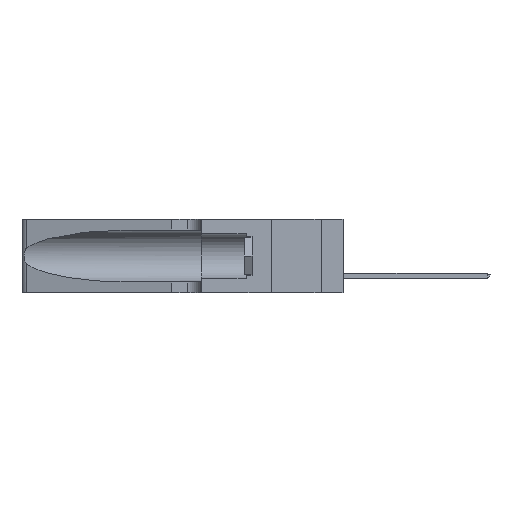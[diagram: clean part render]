
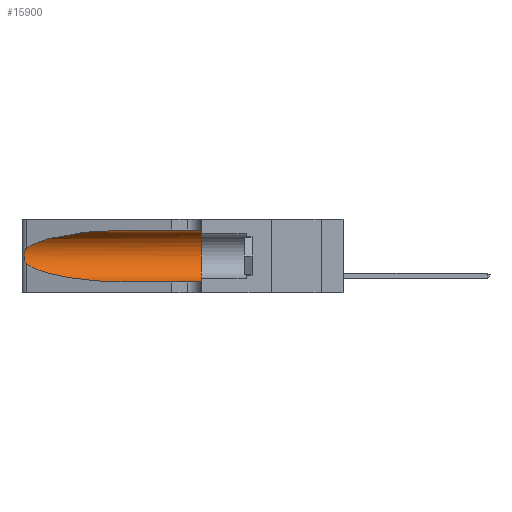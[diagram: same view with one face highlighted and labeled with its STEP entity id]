
A CAD part, left-side view. The second image highlights one B-rep face of the part: STEP entity #15900.
In plain terms, the highlighted cylindrical face has radius 3.308 mm (diameter 6.617 mm), a partial arc.
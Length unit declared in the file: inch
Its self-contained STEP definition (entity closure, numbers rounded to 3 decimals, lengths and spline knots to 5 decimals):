
#396 = CARTESIAN_POINT ( 'NONE',  ( 0.1305, 0.72297, 0.05475 ) ) ;
#763 = CARTESIAN_POINT ( 'NONE',  ( 0.25639, 1.23186, 0.15144 ) ) ;
#1344 = VERTEX_POINT ( 'NONE', #19258 ) ;
#3363 = ORIENTED_EDGE ( 'NONE', *, *, #23458, .F. ) ;
#3405 = CARTESIAN_POINT ( 'NONE',  ( 0.25555, 1.22994, 0.2215 ) ) ;
#3709 = ORIENTED_EDGE ( 'NONE', *, *, #23173, .T. ) ;
#3979 = CARTESIAN_POINT ( 'NONE',  ( 0.26018, 1.23835, 0.19895 ) ) ;
#4084 = CARTESIAN_POINT ( 'NONE',  ( 0.25856, 1.23593, 0.16098 ) ) ;
#5433 = CARTESIAN_POINT ( 'NONE',  ( 0.2373, 1.15595, 0.28018 ) ) ;
#5754 = LINE ( 'NONE', #24213, #10757 ) ;
#6524 = CARTESIAN_POINT ( 'NONE',  ( 0.1305, 0.35, 0.185 ) ) ;
#6635 = ORIENTED_EDGE ( 'NONE', *, *, #16826, .F. ) ;
#6646 = CARTESIAN_POINT ( 'NONE',  ( 0.26075, 1.23896, 0.19203 ) ) ;
#6819 = DIRECTION ( 'NONE',  ( 0., 1., 0. ) ) ;
#7966 = CARTESIAN_POINT ( 'NONE',  ( 0.1305, 1.61858, 0.31525 ) ) ;
#8261 = CARTESIAN_POINT ( 'NONE',  ( 0.25487, 1.22718, 0.14631 ) ) ;
#9195 = ORIENTED_EDGE ( 'NONE', *, *, #22257, .T. ) ;
#10757 = VECTOR ( 'NONE', #29354, 39.37008 ) ;
#12467 =( BOUNDED_CURVE ( )  B_SPLINE_CURVE ( 3, ( #27745, #15193, #5433, #30025 ),
 .UNSPECIFIED., .F., .F. ) 
 B_SPLINE_CURVE_WITH_KNOTS ( ( 4, 4 ),
 ( 1.5708, 2.84003 ),
 .UNSPECIFIED. ) 
 CURVE ( )  GEOMETRIC_REPRESENTATION_ITEM ( )  RATIONAL_B_SPLINE_CURVE ( ( 1., 0.87, 0.87, 1. ) ) 
 REPRESENTATION_ITEM ( '' )  );
#13260 = CARTESIAN_POINT ( 'NONE',  ( 0.2373, 1.15595, 0.08982 ) ) ;
#14399 = EDGE_CURVE ( 'NONE', #31760, #21525, #14988, .T. ) ;
#14880 = CARTESIAN_POINT ( 'NONE',  ( 0.25487, 1.22718, 0.14631 ) ) ;
#14988 =( BOUNDED_CURVE ( )  B_SPLINE_CURVE ( 3, ( #27934, #13260, #20321, #28037 ),
 .UNSPECIFIED., .F., .F. ) 
 B_SPLINE_CURVE_WITH_KNOTS ( ( 4, 4 ),
 ( 3.44316, 4.71239 ),
 .UNSPECIFIED. ) 
 CURVE ( )  GEOMETRIC_REPRESENTATION_ITEM ( )  RATIONAL_B_SPLINE_CURVE ( ( 1., 0.87, 0.87, 1. ) ) 
 REPRESENTATION_ITEM ( '' )  );
#15193 = CARTESIAN_POINT ( 'NONE',  ( 0.18966, 0.96281, 0.31525 ) ) ;
#15900 = ADVANCED_FACE ( 'NONE', ( #16791 ), #21415, .F. ) ;
#16285 = CARTESIAN_POINT ( 'NONE',  ( 0.26017, 1.23833, 0.17102 ) ) ;
#16372 = DIRECTION ( 'NONE',  ( 0., 0., 1. ) ) ;
#16524 = ORIENTED_EDGE ( 'NONE', *, *, #14399, .T. ) ;
#16614 = ORIENTED_EDGE ( 'NONE', *, *, #28576, .T. ) ;
#16791 = FACE_OUTER_BOUND ( 'NONE', #19895, .T. ) ;
#16826 = EDGE_CURVE ( 'NONE', #1344, #20870, #26154, .T. ) ;
#17936 = CARTESIAN_POINT ( 'NONE',  ( 0.1305, 0.35, 0.05475 ) ) ;
#18669 = AXIS2_PLACEMENT_3D ( 'NONE', #19447, #21924, #27036 ) ;
#19258 = CARTESIAN_POINT ( 'NONE',  ( 0.1305, 0.35, 0.31525 ) ) ;
#19447 = CARTESIAN_POINT ( 'NONE',  ( 0.1305, 1.61858, 0.185 ) ) ;
#19895 = EDGE_LOOP ( 'NONE', ( #3709, #16614, #16524, #9195, #6635, #3363 ) ) ;
#20321 = CARTESIAN_POINT ( 'NONE',  ( 0.18966, 0.96281, 0.05475 ) ) ;
#20870 = VERTEX_POINT ( 'NONE', #17936 ) ;
#21415 = CYLINDRICAL_SURFACE ( 'NONE', #18669, 0.13025 ) ;
#21525 = VERTEX_POINT ( 'NONE', #396 ) ;
#21924 = DIRECTION ( 'NONE',  ( 0., -1., 0. ) ) ;
#22257 = EDGE_CURVE ( 'NONE', #21525, #20870, #5754, .T. ) ;
#23054 = CARTESIAN_POINT ( 'NONE',  ( 0.25787, 1.23484, 0.2124 ) ) ;
#23173 = EDGE_CURVE ( 'NONE', #26465, #25362, #12467, .T. ) ;
#23377 = CARTESIAN_POINT ( 'NONE',  ( 0.26075, 1.23896, 0.178 ) ) ;
#23458 = EDGE_CURVE ( 'NONE', #26465, #1344, #29505, .T. ) ;
#24213 = CARTESIAN_POINT ( 'NONE',  ( 0.1305, 1.61858, 0.05475 ) ) ;
#25162 = DIRECTION ( 'NONE',  ( 0., -1., 0. ) ) ;
#25362 = VERTEX_POINT ( 'NONE', #29385 ) ;
#26154 = CIRCLE ( 'NONE', #30618, 0.13025 ) ;
#26362 = CARTESIAN_POINT ( 'NONE',  ( 0.25789, 1.23486, 0.15765 ) ) ;
#26465 = VERTEX_POINT ( 'NONE', #29880 ) ;
#27036 = DIRECTION ( 'NONE',  ( 0., 0., -1. ) ) ;
#27745 = CARTESIAN_POINT ( 'NONE',  ( 0.1305, 0.72297, 0.31525 ) ) ;
#27934 = CARTESIAN_POINT ( 'NONE',  ( 0.25487, 1.22718, 0.14631 ) ) ;
#28037 = CARTESIAN_POINT ( 'NONE',  ( 0.1305, 0.72297, 0.05475 ) ) ;
#28198 = B_SPLINE_CURVE_WITH_KNOTS ( 'NONE', 3,
 ( #30364, #3405, #30134, #23054, #31136, #3979, #6646, #23377, #16285, #4084, #26362, #763, #31665, #14880 ),
 .UNSPECIFIED., .F., .F.,
 ( 4, 2, 2, 2, 2, 2, 4 ),
 ( 0., 0.00027, 0.00053, 0.00107, 0.0016, 0.00187, 0.00214 ),
 .UNSPECIFIED. ) ;
#28576 = EDGE_CURVE ( 'NONE', #25362, #31760, #28198, .T. ) ;
#29354 = DIRECTION ( 'NONE',  ( 0., -1., 0. ) ) ;
#29385 = CARTESIAN_POINT ( 'NONE',  ( 0.25487, 1.22718, 0.22369 ) ) ;
#29505 = LINE ( 'NONE', #7966, #30738 ) ;
#29880 = CARTESIAN_POINT ( 'NONE',  ( 0.1305, 0.72297, 0.31525 ) ) ;
#30025 = CARTESIAN_POINT ( 'NONE',  ( 0.25487, 1.22718, 0.22369 ) ) ;
#30134 = CARTESIAN_POINT ( 'NONE',  ( 0.25639, 1.23184, 0.21858 ) ) ;
#30364 = CARTESIAN_POINT ( 'NONE',  ( 0.25487, 1.22718, 0.22369 ) ) ;
#30618 = AXIS2_PLACEMENT_3D ( 'NONE', #6524, #6819, #16372 ) ;
#30738 = VECTOR ( 'NONE', #25162, 39.37008 ) ;
#31136 = CARTESIAN_POINT ( 'NONE',  ( 0.25854, 1.2359, 0.20912 ) ) ;
#31665 = CARTESIAN_POINT ( 'NONE',  ( 0.25555, 1.22993, 0.14849 ) ) ;
#31760 = VERTEX_POINT ( 'NONE', #8261 ) ;
